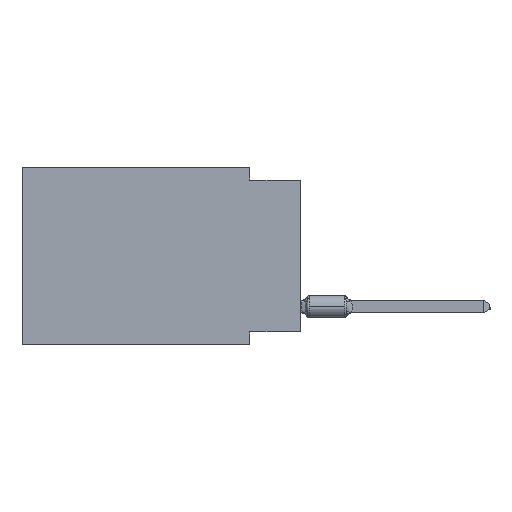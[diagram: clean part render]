
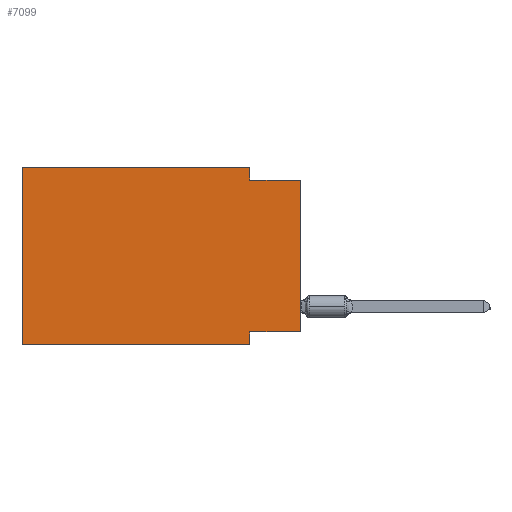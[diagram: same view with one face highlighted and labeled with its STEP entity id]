
A CAD part, left-side view. The second image highlights one B-rep face of the part: STEP entity #7099.
In plain terms, the highlighted planar face has unit normal (-1, 0, 0).
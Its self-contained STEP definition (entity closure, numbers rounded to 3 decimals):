
#1069 = CARTESIAN_POINT ( 'NONE',  ( 0., 2.54, -0.635 ) ) ;
#1775 = CARTESIAN_POINT ( 'NONE',  ( 0., 2.54, -8.89 ) ) ;
#2745 = CARTESIAN_POINT ( 'NONE',  ( 0., 13.97, 0. ) ) ;
#3553 = VERTEX_POINT ( 'NONE', #10699 ) ;
#3587 = ORIENTED_EDGE ( 'NONE', *, *, #7652, .F. ) ;
#5011 = DIRECTION ( 'NONE',  ( 0., 0., -1. ) ) ;
#5093 = VECTOR ( 'NONE', #5011, 1000. ) ;
#5441 = DIRECTION ( 'NONE',  ( 0., 0., 1. ) ) ;
#6068 = EDGE_CURVE ( 'NONE', #3553, #29328, #7362, .T. ) ;
#6576 = CARTESIAN_POINT ( 'NONE',  ( 0., 13.97, -8.89 ) ) ;
#7099 = ADVANCED_FACE ( 'NONE', ( #16901 ), #19587, .F. ) ;
#7176 = LINE ( 'NONE', #30133, #14935 ) ;
#7197 = LINE ( 'NONE', #1775, #29942 ) ;
#7362 = LINE ( 'NONE', #18363, #35413 ) ;
#7652 = EDGE_CURVE ( 'NONE', #19214, #29328, #7176, .T. ) ;
#7654 = DIRECTION ( 'NONE',  ( 0., 0., -1. ) ) ;
#7756 = LINE ( 'NONE', #19872, #15549 ) ;
#7804 = EDGE_CURVE ( 'NONE', #20197, #13797, #7756, .T. ) ;
#8144 = LINE ( 'NONE', #2745, #27210 ) ;
#8445 = DIRECTION ( 'NONE',  ( 0., 1., 0. ) ) ;
#9291 = DIRECTION ( 'NONE',  ( 0., -1., 0. ) ) ;
#10699 = CARTESIAN_POINT ( 'NONE',  ( 0., 0., -8.255 ) ) ;
#10894 = EDGE_CURVE ( 'NONE', #3553, #26281, #23099, .T. ) ;
#11099 = DIRECTION ( 'NONE',  ( 1., 0., 0. ) ) ;
#12350 = DIRECTION ( 'NONE',  ( 0., -1., 0. ) ) ;
#12562 = LINE ( 'NONE', #6576, #23499 ) ;
#12581 = EDGE_CURVE ( 'NONE', #22228, #20197, #8144, .T. ) ;
#12651 = EDGE_CURVE ( 'NONE', #22228, #15622, #12562, .T. ) ;
#13080 = ORIENTED_EDGE ( 'NONE', *, *, #12651, .T. ) ;
#13406 = CARTESIAN_POINT ( 'NONE',  ( 0., 2.54, 0. ) ) ;
#13797 = VERTEX_POINT ( 'NONE', #13406 ) ;
#14935 = VECTOR ( 'NONE', #9291, 1000. ) ;
#15549 = VECTOR ( 'NONE', #31110, 1000. ) ;
#15622 = VERTEX_POINT ( 'NONE', #15786 ) ;
#15786 = CARTESIAN_POINT ( 'NONE',  ( 0., 2.54, -8.89 ) ) ;
#16901 = FACE_OUTER_BOUND ( 'NONE', #21226, .T. ) ;
#18363 = CARTESIAN_POINT ( 'NONE',  ( 0., 0., 0. ) ) ;
#18713 = AXIS2_PLACEMENT_3D ( 'NONE', #28681, #11099, #7654 ) ;
#19127 = DIRECTION ( 'NONE',  ( 0., 0., -1. ) ) ;
#19214 = VERTEX_POINT ( 'NONE', #1069 ) ;
#19587 = PLANE ( 'NONE',  #18713 ) ;
#19641 = CARTESIAN_POINT ( 'NONE',  ( 0., 13.97, -8.89 ) ) ;
#19845 = CARTESIAN_POINT ( 'NONE',  ( 0., 2.54, 0. ) ) ;
#19872 = CARTESIAN_POINT ( 'NONE',  ( 0., 13.97, 0. ) ) ;
#20197 = VERTEX_POINT ( 'NONE', #25366 ) ;
#21195 = VECTOR ( 'NONE', #8445, 1000. ) ;
#21226 = EDGE_LOOP ( 'NONE', ( #37495, #3587, #32087, #34530, #21243, #13080, #33715, #37540 ) ) ;
#21243 = ORIENTED_EDGE ( 'NONE', *, *, #12581, .F. ) ;
#22228 = VERTEX_POINT ( 'NONE', #19641 ) ;
#23099 = LINE ( 'NONE', #37801, #21195 ) ;
#23499 = VECTOR ( 'NONE', #12350, 1000. ) ;
#23652 = CARTESIAN_POINT ( 'NONE',  ( 0., 0., -0.635 ) ) ;
#24151 = DIRECTION ( 'NONE',  ( 0., 0., 1. ) ) ;
#25366 = CARTESIAN_POINT ( 'NONE',  ( 0., 13.97, 0. ) ) ;
#26281 = VERTEX_POINT ( 'NONE', #36580 ) ;
#27210 = VECTOR ( 'NONE', #5441, 1000. ) ;
#28681 = CARTESIAN_POINT ( 'NONE',  ( 0., 13.97, 0. ) ) ;
#29328 = VERTEX_POINT ( 'NONE', #23652 ) ;
#29942 = VECTOR ( 'NONE', #19127, 1000. ) ;
#30133 = CARTESIAN_POINT ( 'NONE',  ( 0., 0., -0.635 ) ) ;
#31110 = DIRECTION ( 'NONE',  ( 0., -1., 0. ) ) ;
#31656 = LINE ( 'NONE', #19845, #5093 ) ;
#32087 = ORIENTED_EDGE ( 'NONE', *, *, #37212, .F. ) ;
#33715 = ORIENTED_EDGE ( 'NONE', *, *, #36719, .F. ) ;
#34530 = ORIENTED_EDGE ( 'NONE', *, *, #7804, .F. ) ;
#35413 = VECTOR ( 'NONE', #24151, 1000. ) ;
#36580 = CARTESIAN_POINT ( 'NONE',  ( 0., 2.54, -8.255 ) ) ;
#36719 = EDGE_CURVE ( 'NONE', #26281, #15622, #7197, .T. ) ;
#37212 = EDGE_CURVE ( 'NONE', #13797, #19214, #31656, .T. ) ;
#37495 = ORIENTED_EDGE ( 'NONE', *, *, #6068, .T. ) ;
#37540 = ORIENTED_EDGE ( 'NONE', *, *, #10894, .F. ) ;
#37801 = CARTESIAN_POINT ( 'NONE',  ( 0., 0., -8.255 ) ) ;
